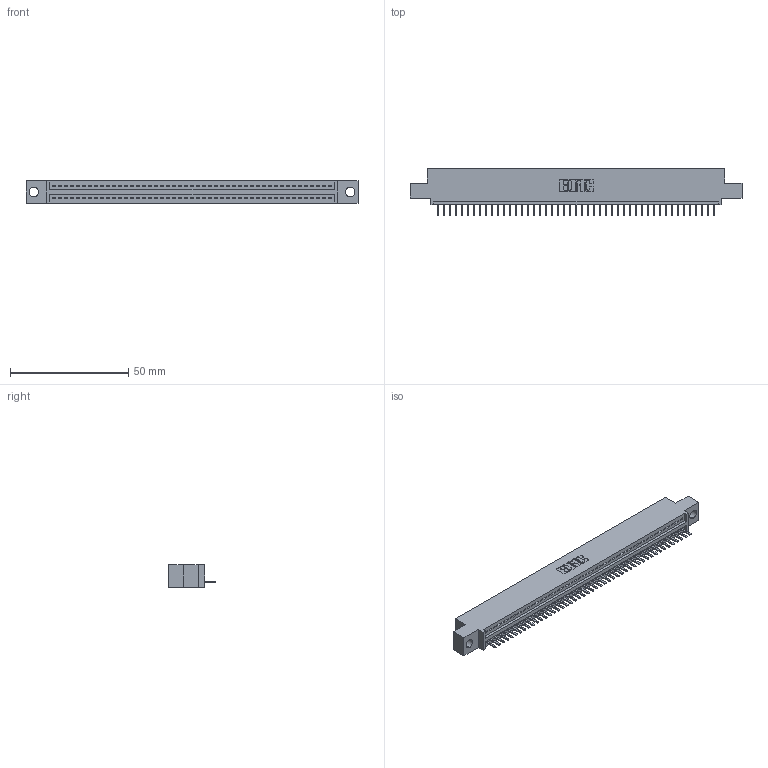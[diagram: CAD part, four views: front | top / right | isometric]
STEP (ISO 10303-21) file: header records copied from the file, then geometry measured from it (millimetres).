
FILE_DESCRIPTION (( 'STEP AP203' ), '1' );
FILE_NAME ('345-047-520-404.STEP', '2018-09-10T08:20:25', ( '' ), ( '' ), 'SwSTEP 2.0', 'SolidWorks 2016', '' );
FILE_SCHEMA (( 'CONFIG_CONTROL_DESIGN' ));
Length unit declared in the file: inch
Products named in the file (3): 345 Part_0.110 Offset - 0.156 Dia-TH; 345-292-001_345-293-120; 345-047-520-404
Assembly tree (48 placements, depth 2):
  345-047-520-404
    345 Part_0.110 Offset - 0.156 Dia-TH
    345-292-001_345-293-120  x47
Bounding box: 140.59 x 19.68 x 9.4 mm (x, y, z)
Volume: 13097.8 mm3; surface area: 16922.1 mm2
Topology: 48 solids, 48 shells, 3044 faces, 9001 edges, 5874 vertices
Faces by surface type: plane 2058, cylinder 986
Entity records: 34949 total; most frequent: CARTESIAN_POINT 6073, ORIENTED_EDGE 6042, DIRECTION 5283, EDGE_CURVE 3021, LINE 2697, VECTOR 2697, VERTEX_POINT 2010, AXIS2_PLACEMENT_3D 1293
